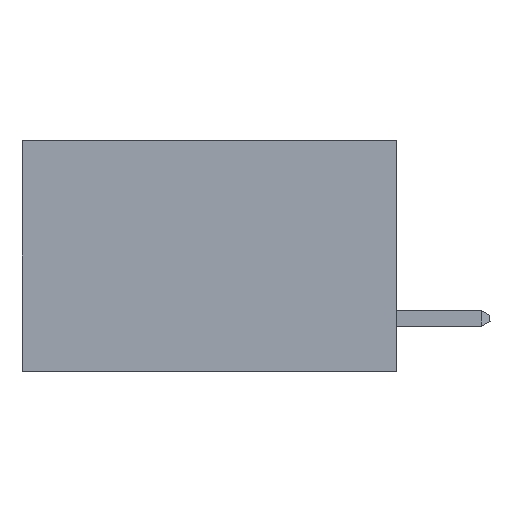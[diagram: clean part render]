
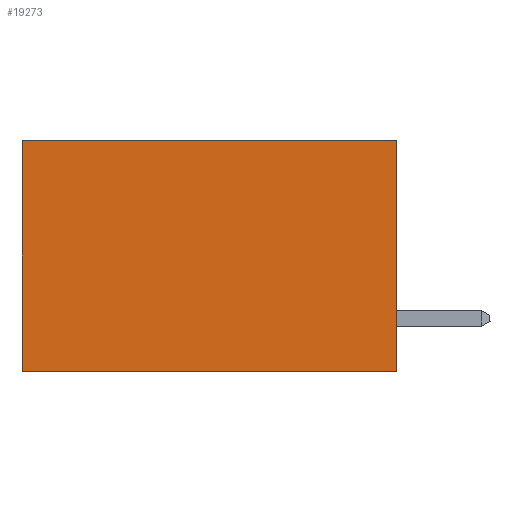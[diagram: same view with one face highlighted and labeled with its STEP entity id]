
A CAD part, left-side view. The second image highlights one B-rep face of the part: STEP entity #19273.
In plain terms, the highlighted planar face has unit normal (-1, 0, 0).
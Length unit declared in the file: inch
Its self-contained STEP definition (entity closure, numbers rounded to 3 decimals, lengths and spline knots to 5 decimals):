
#393 = EDGE_CURVE ( 'NONE', #29702, #4403, #16143, .T. ) ;
#2306 = CARTESIAN_POINT ( 'NONE',  ( 0.298, 0., 0. ) ) ;
#2700 = CARTESIAN_POINT ( 'NONE',  ( 0.298, 0., 0. ) ) ;
#4403 = VERTEX_POINT ( 'NONE', #7237 ) ;
#4583 = VECTOR ( 'NONE', #22179, 39.37008 ) ;
#5189 = DIRECTION ( 'NONE',  ( 0., 0., -1. ) ) ;
#5229 = CARTESIAN_POINT ( 'NONE',  ( 0.298, 0., -0.37 ) ) ;
#6433 = VECTOR ( 'NONE', #9946, 39.37008 ) ;
#7237 = CARTESIAN_POINT ( 'NONE',  ( 0.298, 0.6, -0.37 ) ) ;
#8122 = ORIENTED_EDGE ( 'NONE', *, *, #393, .T. ) ;
#8951 = VERTEX_POINT ( 'NONE', #25026 ) ;
#9946 = DIRECTION ( 'NONE',  ( 0., 1., 0. ) ) ;
#14291 = VECTOR ( 'NONE', #21934, 39.37008 ) ;
#14742 = CARTESIAN_POINT ( 'NONE',  ( 0.298, 0.6, 0. ) ) ;
#16143 = LINE ( 'NONE', #22240, #4583 ) ;
#17023 = AXIS2_PLACEMENT_3D ( 'NONE', #2700, #19895, #5189 ) ;
#18493 = ORIENTED_EDGE ( 'NONE', *, *, #30731, .T. ) ;
#19273 = ADVANCED_FACE ( 'NONE', ( #22173 ), #19789, .F. ) ;
#19789 = PLANE ( 'NONE',  #17023 ) ;
#19895 = DIRECTION ( 'NONE',  ( 1., 0., 0. ) ) ;
#20076 = ORIENTED_EDGE ( 'NONE', *, *, #23350, .F. ) ;
#20430 = EDGE_LOOP ( 'NONE', ( #8122, #20076, #27980, #18493 ) ) ;
#20783 = LINE ( 'NONE', #2306, #14291 ) ;
#21934 = DIRECTION ( 'NONE',  ( 0., 0., -1. ) ) ;
#22125 = VECTOR ( 'NONE', #24068, 39.37008 ) ;
#22173 = FACE_OUTER_BOUND ( 'NONE', #20430, .T. ) ;
#22179 = DIRECTION ( 'NONE',  ( 0., 0., -1. ) ) ;
#22240 = CARTESIAN_POINT ( 'NONE',  ( 0.298, 0.6, 0. ) ) ;
#23350 = EDGE_CURVE ( 'NONE', #28524, #4403, #29282, .T. ) ;
#24068 = DIRECTION ( 'NONE',  ( 0., 1., 0. ) ) ;
#24523 = CARTESIAN_POINT ( 'NONE',  ( 0.298, 0., 0. ) ) ;
#25026 = CARTESIAN_POINT ( 'NONE',  ( 0.298, 0., 0. ) ) ;
#26490 = CARTESIAN_POINT ( 'NONE',  ( 0.298, 0., -0.37 ) ) ;
#26699 = LINE ( 'NONE', #24523, #6433 ) ;
#27980 = ORIENTED_EDGE ( 'NONE', *, *, #28421, .F. ) ;
#28421 = EDGE_CURVE ( 'NONE', #8951, #28524, #20783, .T. ) ;
#28524 = VERTEX_POINT ( 'NONE', #5229 ) ;
#29282 = LINE ( 'NONE', #26490, #22125 ) ;
#29702 = VERTEX_POINT ( 'NONE', #14742 ) ;
#30731 = EDGE_CURVE ( 'NONE', #8951, #29702, #26699, .T. ) ;
